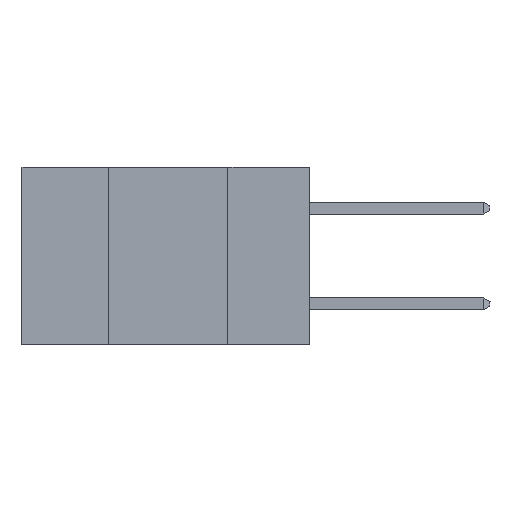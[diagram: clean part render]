
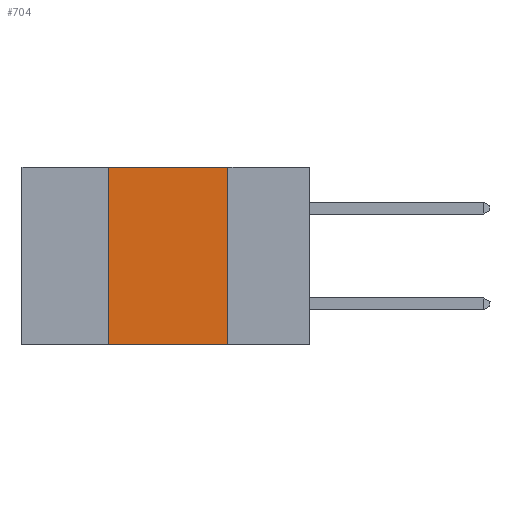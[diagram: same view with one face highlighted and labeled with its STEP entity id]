
A CAD part, left-side view. The second image highlights one B-rep face of the part: STEP entity #704.
In plain terms, the highlighted planar face has unit normal (-1, 0, 0).
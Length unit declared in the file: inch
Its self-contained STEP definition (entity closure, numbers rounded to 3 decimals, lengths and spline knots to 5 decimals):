
#460 = ORIENTED_EDGE ( 'NONE', *, *, #22618, .F. ) ;
#704 = ADVANCED_FACE ( 'NONE', ( #31001 ), #37572, .F. ) ;
#894 = EDGE_CURVE ( 'NONE', #14531, #41670, #32516, .T. ) ;
#1681 = DIRECTION ( 'NONE',  ( 0., 0., 1. ) ) ;
#11324 = LINE ( 'NONE', #41345, #11339 ) ;
#11339 = VECTOR ( 'NONE', #1681, 39.37008 ) ;
#11878 = DIRECTION ( 'NONE',  ( 0., -1., 0. ) ) ;
#12004 = VECTOR ( 'NONE', #11878, 39.37008 ) ;
#12228 = VERTEX_POINT ( 'NONE', #38281 ) ;
#14531 = VERTEX_POINT ( 'NONE', #21872 ) ;
#14810 = AXIS2_PLACEMENT_3D ( 'NONE', #20914, #33846, #34275 ) ;
#15058 = VERTEX_POINT ( 'NONE', #42148 ) ;
#15365 = DIRECTION ( 'NONE',  ( 0., 0., -1. ) ) ;
#15805 = VECTOR ( 'NONE', #15365, 39.37008 ) ;
#17906 = ORIENTED_EDGE ( 'NONE', *, *, #21597, .F. ) ;
#20085 = ORIENTED_EDGE ( 'NONE', *, *, #27714, .F. ) ;
#20914 = CARTESIAN_POINT ( 'NONE',  ( 0., 0.6, 0. ) ) ;
#21597 = EDGE_CURVE ( 'NONE', #14531, #15058, #11324, .T. ) ;
#21872 = CARTESIAN_POINT ( 'NONE',  ( 0., 0.42, -0.37 ) ) ;
#22378 = LINE ( 'NONE', #25881, #12004 ) ;
#22618 = EDGE_CURVE ( 'NONE', #15058, #12228, #22378, .T. ) ;
#25881 = CARTESIAN_POINT ( 'NONE',  ( 0., 0.6, 0. ) ) ;
#27714 = EDGE_CURVE ( 'NONE', #12228, #41670, #35742, .T. ) ;
#29610 = CARTESIAN_POINT ( 'NONE',  ( 0., 0.17, 0. ) ) ;
#31001 = FACE_OUTER_BOUND ( 'NONE', #40271, .T. ) ;
#31249 = ORIENTED_EDGE ( 'NONE', *, *, #894, .T. ) ;
#32516 = LINE ( 'NONE', #35589, #33602 ) ;
#33602 = VECTOR ( 'NONE', #35371, 39.37008 ) ;
#33846 = DIRECTION ( 'NONE',  ( 1., 0., 0. ) ) ;
#34275 = DIRECTION ( 'NONE',  ( 0., 0., -1. ) ) ;
#35371 = DIRECTION ( 'NONE',  ( 0., -1., 0. ) ) ;
#35589 = CARTESIAN_POINT ( 'NONE',  ( 0., 0.6, -0.37 ) ) ;
#35742 = LINE ( 'NONE', #29610, #15805 ) ;
#36617 = CARTESIAN_POINT ( 'NONE',  ( 0., 0.17, -0.37 ) ) ;
#37572 = PLANE ( 'NONE',  #14810 ) ;
#38281 = CARTESIAN_POINT ( 'NONE',  ( 0., 0.17, 0. ) ) ;
#40271 = EDGE_LOOP ( 'NONE', ( #20085, #460, #17906, #31249 ) ) ;
#41345 = CARTESIAN_POINT ( 'NONE',  ( 0., 0.42, 0. ) ) ;
#41670 = VERTEX_POINT ( 'NONE', #36617 ) ;
#42148 = CARTESIAN_POINT ( 'NONE',  ( 0., 0.42, 0. ) ) ;
